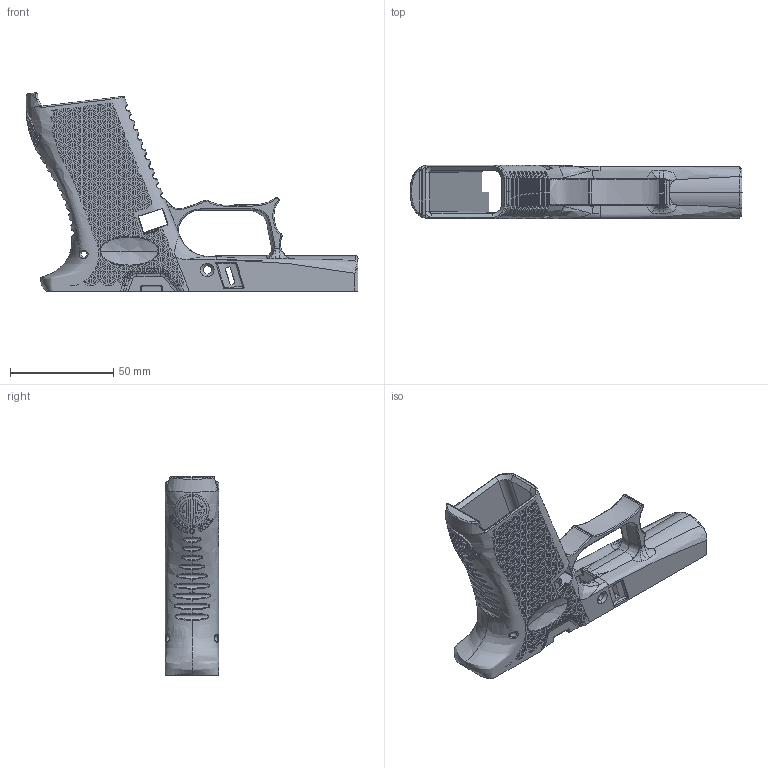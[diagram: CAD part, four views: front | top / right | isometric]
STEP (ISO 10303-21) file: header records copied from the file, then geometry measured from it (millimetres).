
FILE_DESCRIPTION (( 'STEP AP203' ), '1' );
FILE_NAME ('43X Tri-Stipple FDM.STEP', '2020-12-17T02:22:29', ( '' ), ( '' ), 'SwSTEP 2.0', 'SolidWorks 2016', '' );
FILE_SCHEMA (( 'CONFIG_CONTROL_DESIGN' ));
Products named in the file (1): 43X Tri-Stipple FDM
Bounding box: 160.56 x 25.9 x 95.92 mm (x, y, z)
Volume: 61608 mm3; surface area: 44783.9 mm2
Topology: 1 solids, 1 shells, 7020 faces, 18296 edges, 12035 vertices
Faces by surface type: plane 6029, bspline 535, cylinder 416, torus 26, cone 12, sphere 2
Entity records: 263071 total; most frequent: CARTESIAN_POINT 106309, ORIENTED_EDGE 36518, DIRECTION 24687, EDGE_CURVE 18259, VERTEX_POINT 12035, LINE 10595, VECTOR 10595, EDGE_LOOP 7836
